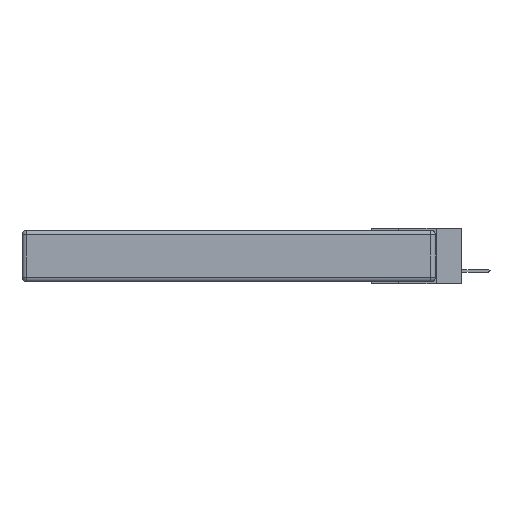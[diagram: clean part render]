
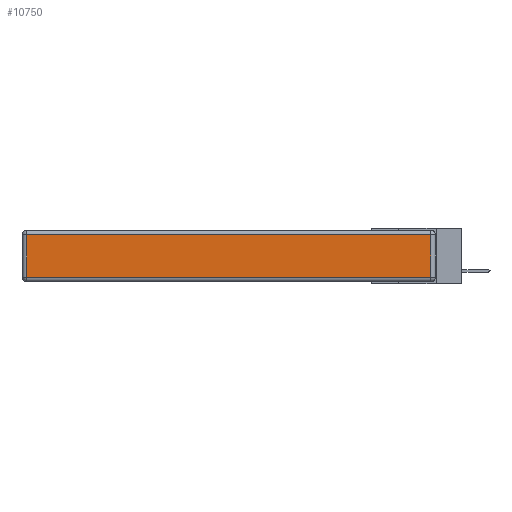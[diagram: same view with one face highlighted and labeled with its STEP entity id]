
A CAD part, left-side view. The second image highlights one B-rep face of the part: STEP entity #10750.
In plain terms, the highlighted planar face has unit normal (-1, 0, 0).
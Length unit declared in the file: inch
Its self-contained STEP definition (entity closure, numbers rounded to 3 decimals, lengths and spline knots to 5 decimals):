
#267 = CARTESIAN_POINT ( 'NONE',  ( 0., 0., -0.313 ) ) ;
#297 = CARTESIAN_POINT ( 'NONE',  ( 0., 2.72, -0.03 ) ) ;
#337 = CARTESIAN_POINT ( 'NONE',  ( 0., 0.03, -0.03 ) ) ;
#480 = LINE ( 'NONE', #10889, #2457 ) ;
#692 = VERTEX_POINT ( 'NONE', #337 ) ;
#1076 = DIRECTION ( 'NONE',  ( 0., 0., 1. ) ) ;
#1223 = ORIENTED_EDGE ( 'NONE', *, *, #1464, .T. ) ;
#1382 = DIRECTION ( 'NONE',  ( 0., 1., 0. ) ) ;
#1464 = EDGE_CURVE ( 'NONE', #17561, #18270, #12980, .T. ) ;
#1680 = VECTOR ( 'NONE', #15761, 39.37008 ) ;
#2131 = VERTEX_POINT ( 'NONE', #297 ) ;
#2143 = CARTESIAN_POINT ( 'NONE',  ( 0., 0.03, -0.313 ) ) ;
#2457 = VECTOR ( 'NONE', #1076, 39.37008 ) ;
#3272 = LINE ( 'NONE', #4626, #6366 ) ;
#4626 = CARTESIAN_POINT ( 'NONE',  ( 0., 2.72, -0.343 ) ) ;
#5161 = EDGE_CURVE ( 'NONE', #18270, #692, #480, .T. ) ;
#5273 = EDGE_CURVE ( 'NONE', #692, #2131, #7925, .T. ) ;
#6366 = VECTOR ( 'NONE', #13035, 39.37008 ) ;
#7407 = FACE_OUTER_BOUND ( 'NONE', #12298, .T. ) ;
#7925 = LINE ( 'NONE', #8527, #15714 ) ;
#8527 = CARTESIAN_POINT ( 'NONE',  ( 0., 2.75, -0.03 ) ) ;
#9189 = ORIENTED_EDGE ( 'NONE', *, *, #5273, .T. ) ;
#10560 = ORIENTED_EDGE ( 'NONE', *, *, #5161, .T. ) ;
#10750 = ADVANCED_FACE ( 'NONE', ( #7407 ), #13617, .T. ) ;
#10889 = CARTESIAN_POINT ( 'NONE',  ( 0., 0.03, -0.343 ) ) ;
#12298 = EDGE_LOOP ( 'NONE', ( #1223, #10560, #9189, #13793 ) ) ;
#12349 = AXIS2_PLACEMENT_3D ( 'NONE', #12490, #12564, #18170 ) ;
#12490 = CARTESIAN_POINT ( 'NONE',  ( 0., 0., -0.343 ) ) ;
#12564 = DIRECTION ( 'NONE',  ( -1., 0., 0. ) ) ;
#12980 = LINE ( 'NONE', #267, #1680 ) ;
#13035 = DIRECTION ( 'NONE',  ( 0., 0., -1. ) ) ;
#13617 = PLANE ( 'NONE',  #12349 ) ;
#13793 = ORIENTED_EDGE ( 'NONE', *, *, #17108, .T. ) ;
#14169 = CARTESIAN_POINT ( 'NONE',  ( 0., 2.72, -0.313 ) ) ;
#15714 = VECTOR ( 'NONE', #1382, 39.37008 ) ;
#15761 = DIRECTION ( 'NONE',  ( 0., -1., 0. ) ) ;
#17108 = EDGE_CURVE ( 'NONE', #2131, #17561, #3272, .T. ) ;
#17561 = VERTEX_POINT ( 'NONE', #14169 ) ;
#18170 = DIRECTION ( 'NONE',  ( 0., 0., 1. ) ) ;
#18270 = VERTEX_POINT ( 'NONE', #2143 ) ;
